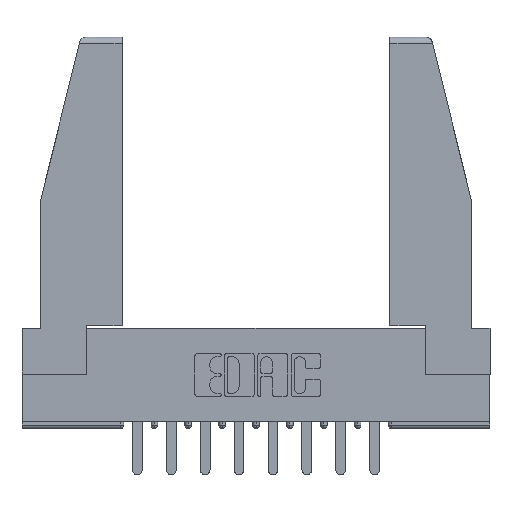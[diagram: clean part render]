
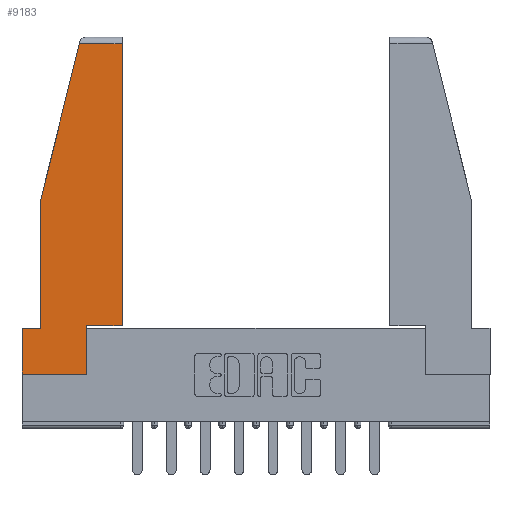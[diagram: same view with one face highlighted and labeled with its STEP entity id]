
A CAD part, top view. The second image highlights one B-rep face of the part: STEP entity #9183.
In plain terms, the highlighted planar face has unit normal (0, 0, 1).
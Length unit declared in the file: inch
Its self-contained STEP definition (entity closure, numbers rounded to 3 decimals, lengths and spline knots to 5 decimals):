
#204 = EDGE_CURVE ( 'NONE', #2261, #2970, #10967, .T. ) ;
#362 = DIRECTION ( 'NONE',  ( 0., 1., 0. ) ) ;
#836 = VECTOR ( 'NONE', #1518, 39.37008 ) ;
#881 = CARTESIAN_POINT ( 'NONE',  ( 0.297, 0.223, 0. ) ) ;
#1066 = DIRECTION ( 'NONE',  ( 0., 1., 0. ) ) ;
#1123 = ORIENTED_EDGE ( 'NONE', *, *, #3238, .T. ) ;
#1198 = VECTOR ( 'NONE', #10334, 39.37008 ) ;
#1229 = ORIENTED_EDGE ( 'NONE', *, *, #8245, .T. ) ;
#1508 = VECTOR ( 'NONE', #1066, 39.37008 ) ;
#1518 = DIRECTION ( 'NONE',  ( -0.239, -0.971, 0. ) ) ;
#1731 = LINE ( 'NONE', #9338, #4460 ) ;
#1928 = EDGE_CURVE ( 'NONE', #7281, #14997, #8730, .T. ) ;
#2122 = LINE ( 'NONE', #10228, #1198 ) ;
#2261 = VERTEX_POINT ( 'NONE', #881 ) ;
#2276 = EDGE_CURVE ( 'NONE', #2548, #8601, #2122, .T. ) ;
#2360 = EDGE_CURVE ( 'NONE', #12529, #2548, #13629, .T. ) ;
#2368 = CARTESIAN_POINT ( 'NONE',  ( 0.086, 0.8, 0. ) ) ;
#2466 = EDGE_LOOP ( 'NONE', ( #8697, #1123, #11722, #5972, #7876, #14960, #13619, #1229, #14964 ) ) ;
#2469 = LINE ( 'NONE', #2368, #14512 ) ;
#2548 = VERTEX_POINT ( 'NONE', #12977 ) ;
#2813 = CARTESIAN_POINT ( 'NONE',  ( 0.461, 0.223, 0. ) ) ;
#2970 = VERTEX_POINT ( 'NONE', #2813 ) ;
#3135 = DIRECTION ( 'NONE',  ( 1., 0., 0. ) ) ;
#3238 = EDGE_CURVE ( 'NONE', #10233, #7281, #1731, .T. ) ;
#3321 = CARTESIAN_POINT ( 'NONE',  ( 0.461, 0.223, 0. ) ) ;
#4088 = EDGE_CURVE ( 'NONE', #2970, #10233, #7909, .T. ) ;
#4337 = VERTEX_POINT ( 'NONE', #6166 ) ;
#4406 = CARTESIAN_POINT ( 'NONE',  ( 0.086, 0.8, 0. ) ) ;
#4460 = VECTOR ( 'NONE', #12840, 39.37008 ) ;
#5853 = CARTESIAN_POINT ( 'NONE',  ( 0.2636, 1.52, 0. ) ) ;
#5972 = ORIENTED_EDGE ( 'NONE', *, *, #7127, .T. ) ;
#6166 = CARTESIAN_POINT ( 'NONE',  ( 0.297, 0., 0. ) ) ;
#6381 = DIRECTION ( 'NONE',  ( 1., 0., 0. ) ) ;
#6488 = LINE ( 'NONE', #7489, #13437 ) ;
#6661 = EDGE_CURVE ( 'NONE', #8601, #4337, #6488, .T. ) ;
#7127 = EDGE_CURVE ( 'NONE', #14997, #12529, #2469, .T. ) ;
#7249 = CARTESIAN_POINT ( 'NONE',  ( 0.297, 0.223, 0. ) ) ;
#7281 = VERTEX_POINT ( 'NONE', #5853 ) ;
#7489 = CARTESIAN_POINT ( 'NONE',  ( 0., 0., 0. ) ) ;
#7876 = ORIENTED_EDGE ( 'NONE', *, *, #2360, .T. ) ;
#7909 = LINE ( 'NONE', #3321, #1508 ) ;
#8245 = EDGE_CURVE ( 'NONE', #4337, #2261, #11558, .T. ) ;
#8601 = VERTEX_POINT ( 'NONE', #14762 ) ;
#8697 = ORIENTED_EDGE ( 'NONE', *, *, #4088, .T. ) ;
#8724 = CARTESIAN_POINT ( 'NONE',  ( 0.297, 0., 0. ) ) ;
#8730 = LINE ( 'NONE', #14348, #836 ) ;
#9013 = VECTOR ( 'NONE', #362, 39.37008 ) ;
#9021 = CARTESIAN_POINT ( 'NONE',  ( 0., 0., 0. ) ) ;
#9183 = ADVANCED_FACE ( 'NONE', ( #9351 ), #12418, .T. ) ;
#9330 = VECTOR ( 'NONE', #11818, 39.37008 ) ;
#9338 = CARTESIAN_POINT ( 'NONE',  ( 0., 1.52, 0. ) ) ;
#9351 = FACE_OUTER_BOUND ( 'NONE', #2466, .T. ) ;
#9484 = CARTESIAN_POINT ( 'NONE',  ( 0.086, 0.21, 0. ) ) ;
#9631 = VECTOR ( 'NONE', #14033, 39.37008 ) ;
#10228 = CARTESIAN_POINT ( 'NONE',  ( 0., 0.21, 0. ) ) ;
#10233 = VERTEX_POINT ( 'NONE', #13357 ) ;
#10253 = DIRECTION ( 'NONE',  ( 0., 0., 1. ) ) ;
#10334 = DIRECTION ( 'NONE',  ( 0., -1., 0. ) ) ;
#10533 = CARTESIAN_POINT ( 'NONE',  ( 0., 0.21, 0. ) ) ;
#10967 = LINE ( 'NONE', #7249, #9330 ) ;
#11558 = LINE ( 'NONE', #8724, #9013 ) ;
#11722 = ORIENTED_EDGE ( 'NONE', *, *, #1928, .T. ) ;
#11818 = DIRECTION ( 'NONE',  ( 1., 0., 0. ) ) ;
#12418 = PLANE ( 'NONE',  #14021 ) ;
#12529 = VERTEX_POINT ( 'NONE', #9484 ) ;
#12840 = DIRECTION ( 'NONE',  ( -1., 0., 0. ) ) ;
#12977 = CARTESIAN_POINT ( 'NONE',  ( 0., 0.21, 0. ) ) ;
#13357 = CARTESIAN_POINT ( 'NONE',  ( 0.461, 1.52, 0. ) ) ;
#13437 = VECTOR ( 'NONE', #6381, 39.37008 ) ;
#13619 = ORIENTED_EDGE ( 'NONE', *, *, #6661, .T. ) ;
#13629 = LINE ( 'NONE', #10533, #9631 ) ;
#14021 = AXIS2_PLACEMENT_3D ( 'NONE', #9021, #10253, #3135 ) ;
#14033 = DIRECTION ( 'NONE',  ( -1., 0., 0. ) ) ;
#14348 = CARTESIAN_POINT ( 'NONE',  ( 0.271, 1.55, 0. ) ) ;
#14512 = VECTOR ( 'NONE', #14699, 39.37008 ) ;
#14699 = DIRECTION ( 'NONE',  ( 0., -1., 0. ) ) ;
#14762 = CARTESIAN_POINT ( 'NONE',  ( 0., 0., 0. ) ) ;
#14960 = ORIENTED_EDGE ( 'NONE', *, *, #2276, .T. ) ;
#14964 = ORIENTED_EDGE ( 'NONE', *, *, #204, .T. ) ;
#14997 = VERTEX_POINT ( 'NONE', #4406 ) ;
